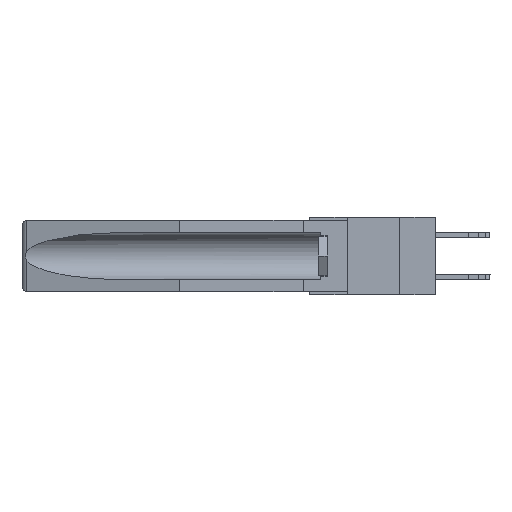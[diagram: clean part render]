
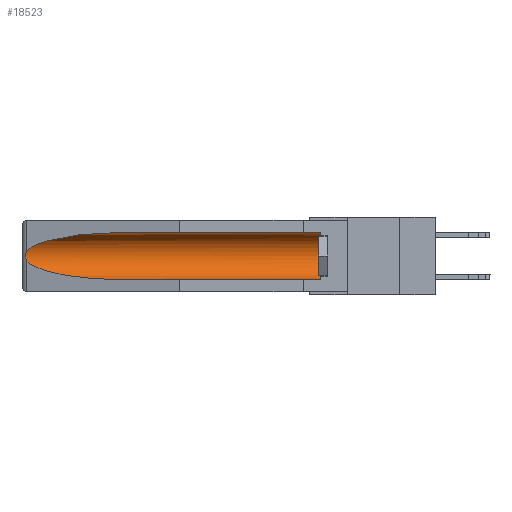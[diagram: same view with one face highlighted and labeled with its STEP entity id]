
A CAD part, left-side view. The second image highlights one B-rep face of the part: STEP entity #18523.
In plain terms, the highlighted cylindrical face has radius 2.857 mm (diameter 5.715 mm), a partial arc.
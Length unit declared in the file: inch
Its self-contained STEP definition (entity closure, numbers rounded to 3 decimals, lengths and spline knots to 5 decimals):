
#182 = LINE ( 'NONE', #703, #1513 ) ;
#265 = CARTESIAN_POINT ( 'NONE',  ( 0.2675, 1.53308, -0.17534 ) ) ;
#703 = CARTESIAN_POINT ( 'NONE',  ( 0.155, -0.30754, -0.059 ) ) ;
#813 = DIRECTION ( 'NONE',  ( 0., 1., 0. ) ) ;
#858 = DIRECTION ( 'NONE',  ( 0., 1., 0. ) ) ;
#885 = CARTESIAN_POINT ( 'NONE',  ( 0.155, 0.126, -0.284 ) ) ;
#899 = CYLINDRICAL_SURFACE ( 'NONE', #18365, 0.1125 ) ;
#1226 = EDGE_CURVE ( 'NONE', #5695, #10533, #18790, .T. ) ;
#1513 = VECTOR ( 'NONE', #858, 39.37008 ) ;
#1654 = ORIENTED_EDGE ( 'NONE', *, *, #12513, .T. ) ;
#2195 = CARTESIAN_POINT ( 'NONE',  ( 0.26597, 1.52961, -0.15275 ) ) ;
#2719 = ORIENTED_EDGE ( 'NONE', *, *, #9414, .T. ) ;
#2906 = CARTESIAN_POINT ( 'NONE',  ( 0.26597, 1.5296, -0.19026 ) ) ;
#3760 = DIRECTION ( 'NONE',  ( 0., 1., 0. ) ) ;
#4081 = CARTESIAN_POINT ( 'NONE',  ( 0.155, 1.07973, -0.284 ) ) ;
#4472 = ORIENTED_EDGE ( 'NONE', *, *, #1226, .T. ) ;
#4800 = CARTESIAN_POINT ( 'NONE',  ( 0.155, 1.07973, -0.059 ) ) ;
#5468 = CARTESIAN_POINT ( 'NONE',  ( 0.26537, 1.52718, -0.14972 ) ) ;
#5612 = CARTESIAN_POINT ( 'NONE',  ( 0.2673, 1.5327, -0.16383 ) ) ;
#5658 = ORIENTED_EDGE ( 'NONE', *, *, #15307, .F. ) ;
#5695 = VERTEX_POINT ( 'NONE', #4800 ) ;
#6389 = FACE_OUTER_BOUND ( 'NONE', #11547, .T. ) ;
#7909 = CARTESIAN_POINT ( 'NONE',  ( 0.155, 1.07973, -0.284 ) ) ;
#8914 = CARTESIAN_POINT ( 'NONE',  ( 0.155, 0.126, -0.059 ) ) ;
#8979 = CARTESIAN_POINT ( 'NONE',  ( 0.26537, 1.52718, -0.19328 ) ) ;
#9163 = CIRCLE ( 'NONE', #16884, 0.1125 ) ;
#9414 = EDGE_CURVE ( 'NONE', #19415, #5695, #182, .T. ) ;
#9782 = ORIENTED_EDGE ( 'NONE', *, *, #16788, .T. ) ;
#10372 = B_SPLINE_CURVE_WITH_KNOTS ( 'NONE', 3,
 ( #12105, #2195, #15514, #5612, #18899, #265, #12460, #20615, #2906, #14475 ),
 .UNSPECIFIED., .F., .F.,
 ( 4, 2, 2, 2, 4 ),
 ( 0., 0.00029, 0.00058, 0.00087, 0.00117 ),
 .UNSPECIFIED. ) ;
#10533 = VERTEX_POINT ( 'NONE', #5468 ) ;
#11547 = EDGE_LOOP ( 'NONE', ( #4472, #9782, #15124, #5658, #1654, #2719 ) ) ;
#12105 = CARTESIAN_POINT ( 'NONE',  ( 0.26537, 1.52718, -0.14972 ) ) ;
#12378 = EDGE_CURVE ( 'NONE', #15320, #21330, #18512, .T. ) ;
#12460 = CARTESIAN_POINT ( 'NONE',  ( 0.2673, 1.53269, -0.17917 ) ) ;
#12513 = EDGE_CURVE ( 'NONE', #15293, #19415, #9163, .T. ) ;
#12546 = CARTESIAN_POINT ( 'NONE',  ( 0.25451, 1.48313, -0.24835 ) ) ;
#12660 = DIRECTION ( 'NONE',  ( 0., -1., 0. ) ) ;
#12738 = DIRECTION ( 'NONE',  ( 0., 0., 1. ) ) ;
#13752 = VECTOR ( 'NONE', #813, 39.37008 ) ;
#14226 = CARTESIAN_POINT ( 'NONE',  ( 0.21114, 1.30732, -0.284 ) ) ;
#14475 = CARTESIAN_POINT ( 'NONE',  ( 0.26537, 1.52718, -0.19328 ) ) ;
#14662 = DIRECTION ( 'NONE',  ( 0., 0., 1. ) ) ;
#15124 = ORIENTED_EDGE ( 'NONE', *, *, #12378, .T. ) ;
#15293 = VERTEX_POINT ( 'NONE', #885 ) ;
#15307 = EDGE_CURVE ( 'NONE', #15293, #21330, #17520, .T. ) ;
#15320 = VERTEX_POINT ( 'NONE', #20925 ) ;
#15514 = CARTESIAN_POINT ( 'NONE',  ( 0.26654, 1.53092, -0.15636 ) ) ;
#16788 = EDGE_CURVE ( 'NONE', #10533, #15320, #10372, .T. ) ;
#16884 = AXIS2_PLACEMENT_3D ( 'NONE', #19312, #12660, #12738 ) ;
#17169 = CARTESIAN_POINT ( 'NONE',  ( 0.155, 1.07973, -0.059 ) ) ;
#17222 = CARTESIAN_POINT ( 'NONE',  ( 0.155, -0.30754, -0.1715 ) ) ;
#17248 = CARTESIAN_POINT ( 'NONE',  ( 0.21114, 1.30732, -0.059 ) ) ;
#17310 = CARTESIAN_POINT ( 'NONE',  ( 0.26537, 1.52718, -0.14972 ) ) ;
#17520 = LINE ( 'NONE', #19359, #13752 ) ;
#18365 = AXIS2_PLACEMENT_3D ( 'NONE', #17222, #3760, #14662 ) ;
#18512 =( BOUNDED_CURVE ( )  B_SPLINE_CURVE ( 3, ( #8979, #12546, #14226, #4081 ),
 .UNSPECIFIED., .F., .F. ) 
 B_SPLINE_CURVE_WITH_KNOTS ( ( 4, 4 ),
 ( 0.1948, 1.5708 ),
 .UNSPECIFIED. ) 
 CURVE ( )  GEOMETRIC_REPRESENTATION_ITEM ( )  RATIONAL_B_SPLINE_CURVE ( ( 1., 0.848, 0.848, 1. ) ) 
 REPRESENTATION_ITEM ( '' )  );
#18523 = ADVANCED_FACE ( 'NONE', ( #6389 ), #899, .F. ) ;
#18790 =( BOUNDED_CURVE ( )  B_SPLINE_CURVE ( 3, ( #17169, #17248, #19019, #17310 ),
 .UNSPECIFIED., .F., .F. ) 
 B_SPLINE_CURVE_WITH_KNOTS ( ( 4, 4 ),
 ( 4.71239, 6.08839 ),
 .UNSPECIFIED. ) 
 CURVE ( )  GEOMETRIC_REPRESENTATION_ITEM ( )  RATIONAL_B_SPLINE_CURVE ( ( 1., 0.848, 0.848, 1. ) ) 
 REPRESENTATION_ITEM ( '' )  );
#18899 = CARTESIAN_POINT ( 'NONE',  ( 0.2675, 1.53308, -0.16763 ) ) ;
#19019 = CARTESIAN_POINT ( 'NONE',  ( 0.25451, 1.48313, -0.09465 ) ) ;
#19312 = CARTESIAN_POINT ( 'NONE',  ( 0.155, 0.126, -0.1715 ) ) ;
#19359 = CARTESIAN_POINT ( 'NONE',  ( 0.155, -0.30754, -0.284 ) ) ;
#19415 = VERTEX_POINT ( 'NONE', #8914 ) ;
#20615 = CARTESIAN_POINT ( 'NONE',  ( 0.26655, 1.53094, -0.18657 ) ) ;
#20925 = CARTESIAN_POINT ( 'NONE',  ( 0.26537, 1.52718, -0.19328 ) ) ;
#21330 = VERTEX_POINT ( 'NONE', #7909 ) ;
